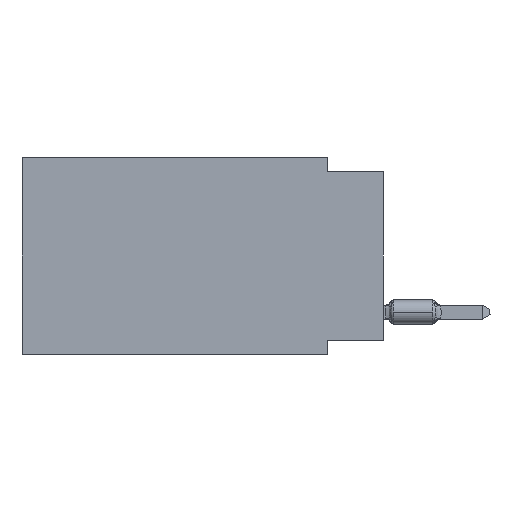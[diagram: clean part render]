
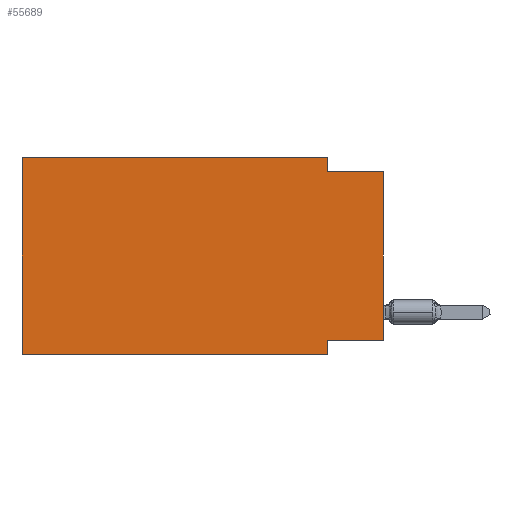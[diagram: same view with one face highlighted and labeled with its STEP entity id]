
A CAD part, left-side view. The second image highlights one B-rep face of the part: STEP entity #55689.
In plain terms, the highlighted planar face has unit normal (-1, 0, 0).
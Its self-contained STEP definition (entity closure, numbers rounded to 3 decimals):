
#1142 = DIRECTION ( 'NONE',  ( 0., -1., 0. ) ) ;
#3700 = CARTESIAN_POINT ( 'NONE',  ( 0., 2.54, -8.89 ) ) ;
#6229 = ORIENTED_EDGE ( 'NONE', *, *, #53021, .F. ) ;
#6697 = VERTEX_POINT ( 'NONE', #29429 ) ;
#6706 = CARTESIAN_POINT ( 'NONE',  ( 0., 16.383, -8.89 ) ) ;
#6895 = DIRECTION ( 'NONE',  ( 0., 0., 1. ) ) ;
#8539 = EDGE_CURVE ( 'NONE', #53812, #47437, #59484, .T. ) ;
#8813 = CARTESIAN_POINT ( 'NONE',  ( 0., 0., 0. ) ) ;
#9309 = AXIS2_PLACEMENT_3D ( 'NONE', #35241, #49610, #54596 ) ;
#9852 = LINE ( 'NONE', #3700, #37036 ) ;
#9915 = EDGE_CURVE ( 'NONE', #35501, #6697, #29262, .T. ) ;
#11163 = CARTESIAN_POINT ( 'NONE',  ( 0., 0., -0.635 ) ) ;
#12285 = DIRECTION ( 'NONE',  ( 0., -1., 0. ) ) ;
#14026 = VECTOR ( 'NONE', #20208, 1000. ) ;
#14056 = CARTESIAN_POINT ( 'NONE',  ( 0., 16.383, -8.89 ) ) ;
#14586 = CARTESIAN_POINT ( 'NONE',  ( 0., 2.54, 0. ) ) ;
#15304 = EDGE_CURVE ( 'NONE', #6697, #28414, #19590, .T. ) ;
#16175 = PLANE ( 'NONE',  #9309 ) ;
#17292 = VECTOR ( 'NONE', #6895, 1000. ) ;
#17571 = DIRECTION ( 'NONE',  ( 0., 0., 1. ) ) ;
#17860 = LINE ( 'NONE', #8813, #61219 ) ;
#18171 = CARTESIAN_POINT ( 'NONE',  ( 0., 2.54, -0.635 ) ) ;
#19590 = LINE ( 'NONE', #14586, #14026 ) ;
#19921 = CARTESIAN_POINT ( 'NONE',  ( 0., 16.383, 0. ) ) ;
#20208 = DIRECTION ( 'NONE',  ( 0., 0., -1. ) ) ;
#24658 = ORIENTED_EDGE ( 'NONE', *, *, #28375, .T. ) ;
#25849 = CARTESIAN_POINT ( 'NONE',  ( 0., 2.54, -8.89 ) ) ;
#26002 = ORIENTED_EDGE ( 'NONE', *, *, #44349, .F. ) ;
#26270 = EDGE_LOOP ( 'NONE', ( #24658, #26002, #51710, #31054, #53995, #49804, #6229, #39095 ) ) ;
#28375 = EDGE_CURVE ( 'NONE', #35725, #34025, #17860, .T. ) ;
#28411 = VECTOR ( 'NONE', #1142, 1000. ) ;
#28414 = VERTEX_POINT ( 'NONE', #18171 ) ;
#28663 = EDGE_CURVE ( 'NONE', #53812, #35501, #58459, .T. ) ;
#29262 = LINE ( 'NONE', #48643, #28411 ) ;
#29429 = CARTESIAN_POINT ( 'NONE',  ( 0., 2.54, 0. ) ) ;
#31054 = ORIENTED_EDGE ( 'NONE', *, *, #9915, .F. ) ;
#31075 = DIRECTION ( 'NONE',  ( 0., -1., 0. ) ) ;
#34025 = VERTEX_POINT ( 'NONE', #11163 ) ;
#34713 = CARTESIAN_POINT ( 'NONE',  ( 0., 16.383, 0. ) ) ;
#35241 = CARTESIAN_POINT ( 'NONE',  ( 0., 16.383, 0. ) ) ;
#35501 = VERTEX_POINT ( 'NONE', #19921 ) ;
#35725 = VERTEX_POINT ( 'NONE', #60196 ) ;
#37036 = VECTOR ( 'NONE', #41512, 1000. ) ;
#37542 = CARTESIAN_POINT ( 'NONE',  ( 0., 2.54, -8.255 ) ) ;
#38750 = LINE ( 'NONE', #47197, #47986 ) ;
#39095 = ORIENTED_EDGE ( 'NONE', *, *, #45731, .F. ) ;
#39628 = FACE_OUTER_BOUND ( 'NONE', #26270, .T. ) ;
#41512 = DIRECTION ( 'NONE',  ( 0., 0., -1. ) ) ;
#43804 = VECTOR ( 'NONE', #12285, 1000. ) ;
#44349 = EDGE_CURVE ( 'NONE', #28414, #34025, #50748, .T. ) ;
#44933 = VERTEX_POINT ( 'NONE', #37542 ) ;
#45468 = CARTESIAN_POINT ( 'NONE',  ( 0., 0., -0.635 ) ) ;
#45731 = EDGE_CURVE ( 'NONE', #35725, #44933, #38750, .T. ) ;
#47197 = CARTESIAN_POINT ( 'NONE',  ( 0., 0., -8.255 ) ) ;
#47437 = VERTEX_POINT ( 'NONE', #25849 ) ;
#47986 = VECTOR ( 'NONE', #52190, 1000. ) ;
#48643 = CARTESIAN_POINT ( 'NONE',  ( 0., 16.383, 0. ) ) ;
#49610 = DIRECTION ( 'NONE',  ( 1., 0., 0. ) ) ;
#49804 = ORIENTED_EDGE ( 'NONE', *, *, #8539, .T. ) ;
#50748 = LINE ( 'NONE', #45468, #58969 ) ;
#51710 = ORIENTED_EDGE ( 'NONE', *, *, #15304, .F. ) ;
#52190 = DIRECTION ( 'NONE',  ( 0., 1., 0. ) ) ;
#53021 = EDGE_CURVE ( 'NONE', #44933, #47437, #9852, .T. ) ;
#53812 = VERTEX_POINT ( 'NONE', #14056 ) ;
#53995 = ORIENTED_EDGE ( 'NONE', *, *, #28663, .F. ) ;
#54596 = DIRECTION ( 'NONE',  ( 0., 0., -1. ) ) ;
#55689 = ADVANCED_FACE ( 'NONE', ( #39628 ), #16175, .F. ) ;
#58459 = LINE ( 'NONE', #34713, #17292 ) ;
#58969 = VECTOR ( 'NONE', #31075, 1000. ) ;
#59484 = LINE ( 'NONE', #6706, #43804 ) ;
#60196 = CARTESIAN_POINT ( 'NONE',  ( 0., 0., -8.255 ) ) ;
#61219 = VECTOR ( 'NONE', #17571, 1000. ) ;
